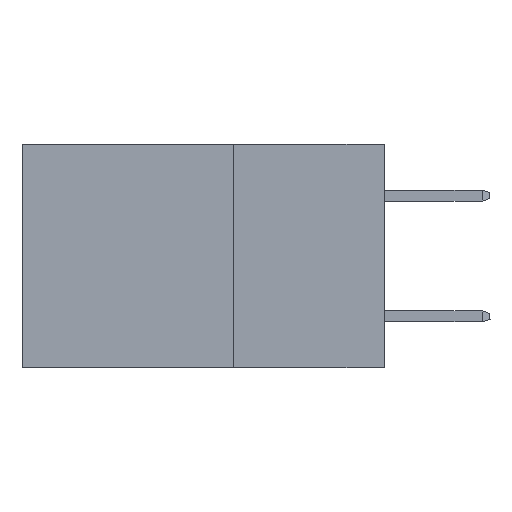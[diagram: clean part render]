
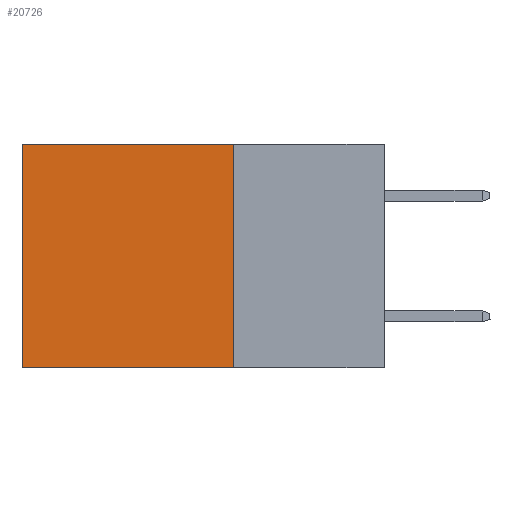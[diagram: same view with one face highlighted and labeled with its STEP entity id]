
A CAD part, left-side view. The second image highlights one B-rep face of the part: STEP entity #20726.
In plain terms, the highlighted planar face has unit normal (-1, 0, 0).
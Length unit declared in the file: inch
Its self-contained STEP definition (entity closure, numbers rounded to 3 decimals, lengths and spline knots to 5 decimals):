
#594 = CARTESIAN_POINT ( 'NONE',  ( 0.2615, 0.25, -0.37 ) ) ;
#1621 = CARTESIAN_POINT ( 'NONE',  ( 0.2615, 0.25, 0. ) ) ;
#1804 = CARTESIAN_POINT ( 'NONE',  ( 0.2615, 0.25, -0.37 ) ) ;
#1922 = VERTEX_POINT ( 'NONE', #13619 ) ;
#2311 = CARTESIAN_POINT ( 'NONE',  ( 0.2615, 0.25, -0.37 ) ) ;
#3249 = DIRECTION ( 'NONE',  ( 0., 1., 0. ) ) ;
#3452 = LINE ( 'NONE', #1621, #18185 ) ;
#4434 = CARTESIAN_POINT ( 'NONE',  ( 0.2615, 0.25, 0. ) ) ;
#6010 = VERTEX_POINT ( 'NONE', #13335 ) ;
#6079 = VERTEX_POINT ( 'NONE', #4434 ) ;
#7209 = ORIENTED_EDGE ( 'NONE', *, *, #10294, .T. ) ;
#7447 = AXIS2_PLACEMENT_3D ( 'NONE', #9363, #20569, #10971 ) ;
#9246 = LINE ( 'NONE', #10793, #17340 ) ;
#9363 = CARTESIAN_POINT ( 'NONE',  ( 0.2615, 0.25, -0.37 ) ) ;
#10294 = EDGE_CURVE ( 'NONE', #6079, #6010, #3452, .T. ) ;
#10532 = EDGE_CURVE ( 'NONE', #6079, #12621, #14152, .T. ) ;
#10736 = LINE ( 'NONE', #2311, #18319 ) ;
#10793 = CARTESIAN_POINT ( 'NONE',  ( 0.2615, 0.6, -0.37 ) ) ;
#10862 = DIRECTION ( 'NONE',  ( 0., 0., -1. ) ) ;
#10971 = DIRECTION ( 'NONE',  ( 0., 0., -1. ) ) ;
#12297 = EDGE_CURVE ( 'NONE', #6010, #1922, #9246, .T. ) ;
#12621 = VERTEX_POINT ( 'NONE', #1804 ) ;
#12832 = ORIENTED_EDGE ( 'NONE', *, *, #10532, .F. ) ;
#13335 = CARTESIAN_POINT ( 'NONE',  ( 0.2615, 0.6, 0. ) ) ;
#13619 = CARTESIAN_POINT ( 'NONE',  ( 0.2615, 0.6, -0.37 ) ) ;
#13655 = VECTOR ( 'NONE', #15284, 39.37008 ) ;
#14152 = LINE ( 'NONE', #594, #13655 ) ;
#15010 = FACE_OUTER_BOUND ( 'NONE', #15052, .T. ) ;
#15052 = EDGE_LOOP ( 'NONE', ( #15582, #16120, #12832, #7209 ) ) ;
#15284 = DIRECTION ( 'NONE',  ( 0., 0., -1. ) ) ;
#15349 = DIRECTION ( 'NONE',  ( 0., 1., 0. ) ) ;
#15582 = ORIENTED_EDGE ( 'NONE', *, *, #12297, .T. ) ;
#16120 = ORIENTED_EDGE ( 'NONE', *, *, #19834, .F. ) ;
#17340 = VECTOR ( 'NONE', #10862, 39.37008 ) ;
#18185 = VECTOR ( 'NONE', #3249, 39.37008 ) ;
#18319 = VECTOR ( 'NONE', #15349, 39.37008 ) ;
#18991 = PLANE ( 'NONE',  #7447 ) ;
#19834 = EDGE_CURVE ( 'NONE', #12621, #1922, #10736, .T. ) ;
#20569 = DIRECTION ( 'NONE',  ( 1., 0., 0. ) ) ;
#20726 = ADVANCED_FACE ( 'NONE', ( #15010 ), #18991, .F. ) ;
